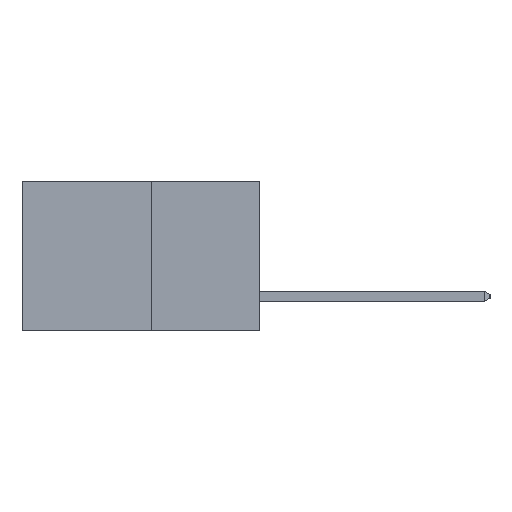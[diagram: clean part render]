
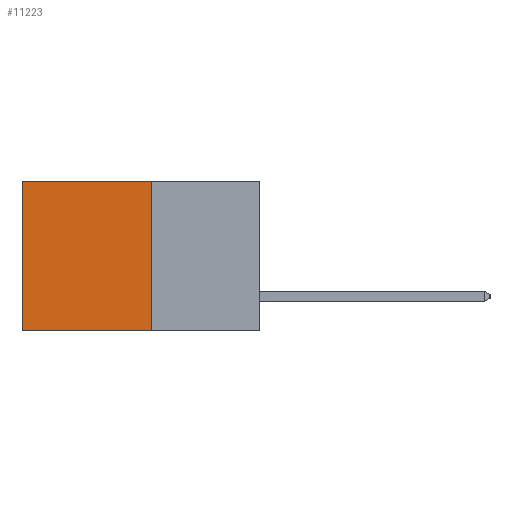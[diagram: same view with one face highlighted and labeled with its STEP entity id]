
A CAD part, left-side view. The second image highlights one B-rep face of the part: STEP entity #11223.
In plain terms, the highlighted planar face has unit normal (-1, 0, 0).
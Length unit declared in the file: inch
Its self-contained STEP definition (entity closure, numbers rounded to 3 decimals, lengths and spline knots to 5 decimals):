
#199 = ORIENTED_EDGE ( 'NONE', *, *, #5563, .T. ) ;
#692 = VECTOR ( 'NONE', #11409, 39.37008 ) ;
#1294 = CARTESIAN_POINT ( 'NONE',  ( 0.277, 0.27, 0. ) ) ;
#1461 = ORIENTED_EDGE ( 'NONE', *, *, #6510, .T. ) ;
#1513 = VECTOR ( 'NONE', #16132, 39.37008 ) ;
#2804 = ORIENTED_EDGE ( 'NONE', *, *, #5243, .F. ) ;
#3538 = CARTESIAN_POINT ( 'NONE',  ( 0.277, 0.59, 0. ) ) ;
#4256 = DIRECTION ( 'NONE',  ( 0., 0., -1. ) ) ;
#5243 = EDGE_CURVE ( 'NONE', #20704, #7023, #10485, .T. ) ;
#5563 = EDGE_CURVE ( 'NONE', #18654, #12233, #8638, .T. ) ;
#6510 = EDGE_CURVE ( 'NONE', #12233, #7023, #10953, .T. ) ;
#6644 = EDGE_CURVE ( 'NONE', #18654, #20704, #12815, .T. ) ;
#7023 = VERTEX_POINT ( 'NONE', #21569 ) ;
#8327 = VECTOR ( 'NONE', #12644, 39.37008 ) ;
#8638 = LINE ( 'NONE', #11355, #692 ) ;
#10321 = FACE_OUTER_BOUND ( 'NONE', #14075, .T. ) ;
#10485 = LINE ( 'NONE', #16153, #1513 ) ;
#10953 = LINE ( 'NONE', #16477, #15345 ) ;
#11223 = ADVANCED_FACE ( 'NONE', ( #10321 ), #12664, .F. ) ;
#11355 = CARTESIAN_POINT ( 'NONE',  ( 0.277, 0.27, 0. ) ) ;
#11409 = DIRECTION ( 'NONE',  ( 0., 1., 0. ) ) ;
#12233 = VERTEX_POINT ( 'NONE', #3538 ) ;
#12319 = CARTESIAN_POINT ( 'NONE',  ( 0.277, 0.27, -0.37 ) ) ;
#12644 = DIRECTION ( 'NONE',  ( 0., 0., -1. ) ) ;
#12664 = PLANE ( 'NONE',  #20822 ) ;
#12815 = LINE ( 'NONE', #12319, #8327 ) ;
#14075 = EDGE_LOOP ( 'NONE', ( #1461, #2804, #17786, #199 ) ) ;
#14287 = DIRECTION ( 'NONE',  ( 1., 0., 0. ) ) ;
#15345 = VECTOR ( 'NONE', #16797, 39.37008 ) ;
#16132 = DIRECTION ( 'NONE',  ( 0., 1., 0. ) ) ;
#16153 = CARTESIAN_POINT ( 'NONE',  ( 0.277, 0.27, -0.37 ) ) ;
#16477 = CARTESIAN_POINT ( 'NONE',  ( 0.277, 0.59, -0.37 ) ) ;
#16543 = CARTESIAN_POINT ( 'NONE',  ( 0.277, 0.27, -0.37 ) ) ;
#16797 = DIRECTION ( 'NONE',  ( 0., 0., -1. ) ) ;
#17786 = ORIENTED_EDGE ( 'NONE', *, *, #6644, .F. ) ;
#18654 = VERTEX_POINT ( 'NONE', #1294 ) ;
#19267 = CARTESIAN_POINT ( 'NONE',  ( 0.277, 0.27, -0.37 ) ) ;
#20704 = VERTEX_POINT ( 'NONE', #16543 ) ;
#20822 = AXIS2_PLACEMENT_3D ( 'NONE', #19267, #14287, #4256 ) ;
#21569 = CARTESIAN_POINT ( 'NONE',  ( 0.277, 0.59, -0.37 ) ) ;
